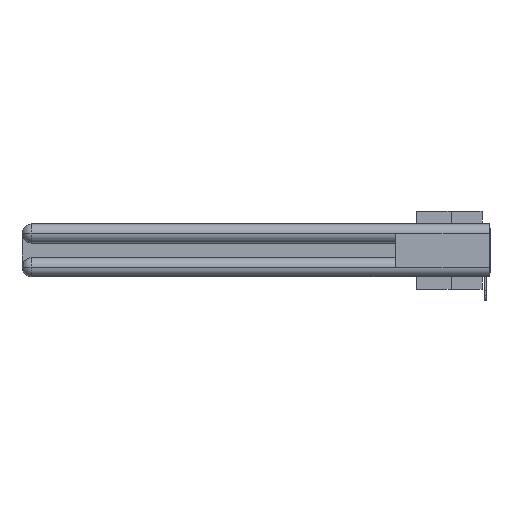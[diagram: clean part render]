
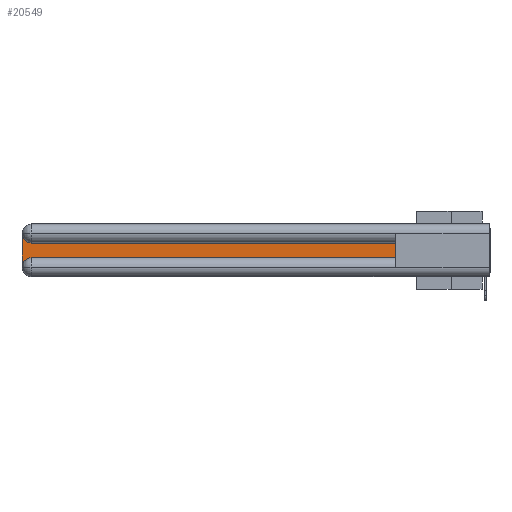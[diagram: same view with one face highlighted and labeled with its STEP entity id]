
A CAD part, left-side view. The second image highlights one B-rep face of the part: STEP entity #20549.
In plain terms, the highlighted planar face has unit normal (-1, 0, 0).
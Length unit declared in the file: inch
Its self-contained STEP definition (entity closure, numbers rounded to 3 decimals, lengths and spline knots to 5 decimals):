
#40 = ORIENTED_EDGE ( 'NONE', *, *, #15962, .T. ) ;
#512 = ORIENTED_EDGE ( 'NONE', *, *, #20141, .T. ) ;
#1826 = VECTOR ( 'NONE', #13648, 39.37008 ) ;
#1877 = DIRECTION ( 'NONE',  ( 1., 0., 0. ) ) ;
#3248 = ORIENTED_EDGE ( 'NONE', *, *, #32857, .T. ) ;
#4267 = VERTEX_POINT ( 'NONE', #34073 ) ;
#5395 = VERTEX_POINT ( 'NONE', #25732 ) ;
#6760 = VECTOR ( 'NONE', #33161, 39.37008 ) ;
#7041 = CARTESIAN_POINT ( 'NONE',  ( 0.075, 0.6, -0.2175 ) ) ;
#7051 = DIRECTION ( 'NONE',  ( 0., -1., 0. ) ) ;
#7186 = CARTESIAN_POINT ( 'NONE',  ( 0.075, 2.94, -0.0625 ) ) ;
#7679 = CARTESIAN_POINT ( 'NONE',  ( 0.075, 2.94, -0.1225 ) ) ;
#9312 = FACE_OUTER_BOUND ( 'NONE', #15956, .T. ) ;
#9491 = DIRECTION ( 'NONE',  ( 1., 0., 0. ) ) ;
#10404 = VECTOR ( 'NONE', #7051, 39.37008 ) ;
#10485 = AXIS2_PLACEMENT_3D ( 'NONE', #7186, #28035, #20163 ) ;
#11069 = EDGE_CURVE ( 'NONE', #18646, #5395, #17308, .T. ) ;
#13648 = DIRECTION ( 'NONE',  ( 0., 0., -1. ) ) ;
#15139 = CARTESIAN_POINT ( 'NONE',  ( 0.075, 3., -0.1225 ) ) ;
#15451 = VERTEX_POINT ( 'NONE', #31141 ) ;
#15563 = ORIENTED_EDGE ( 'NONE', *, *, #25791, .T. ) ;
#15956 = EDGE_LOOP ( 'NONE', ( #40, #26945, #512, #24864, #15563, #3248 ) ) ;
#15962 = EDGE_CURVE ( 'NONE', #15451, #18646, #18774, .T. ) ;
#17091 = CARTESIAN_POINT ( 'NONE',  ( 0.075, 3., -0.2775 ) ) ;
#17308 = CIRCLE ( 'NONE', #10485, 0.06 ) ;
#17358 = AXIS2_PLACEMENT_3D ( 'NONE', #15139, #1877, #26023 ) ;
#18629 = CARTESIAN_POINT ( 'NONE',  ( 0.075, 3., -0.2175 ) ) ;
#18646 = VERTEX_POINT ( 'NONE', #7679 ) ;
#18774 = LINE ( 'NONE', #28077, #30385 ) ;
#18946 = AXIS2_PLACEMENT_3D ( 'NONE', #25382, #9491, #30683 ) ;
#20141 = EDGE_CURVE ( 'NONE', #5395, #33475, #23021, .T. ) ;
#20163 = DIRECTION ( 'NONE',  ( 0., 0., -1. ) ) ;
#20549 = ADVANCED_FACE ( 'NONE', ( #9312 ), #31017, .F. ) ;
#23021 = LINE ( 'NONE', #18629, #1826 ) ;
#23280 = CARTESIAN_POINT ( 'NONE',  ( 0.075, 0.6, -0.2175 ) ) ;
#23400 = EDGE_CURVE ( 'NONE', #33475, #32467, #31752, .T. ) ;
#24864 = ORIENTED_EDGE ( 'NONE', *, *, #23400, .T. ) ;
#25382 = CARTESIAN_POINT ( 'NONE',  ( 0.075, 2.94, -0.2775 ) ) ;
#25732 = CARTESIAN_POINT ( 'NONE',  ( 0.075, 3., -0.0625 ) ) ;
#25791 = EDGE_CURVE ( 'NONE', #32467, #4267, #27818, .T. ) ;
#26023 = DIRECTION ( 'NONE',  ( 0., 0., -1. ) ) ;
#26945 = ORIENTED_EDGE ( 'NONE', *, *, #11069, .T. ) ;
#27818 = LINE ( 'NONE', #23280, #10404 ) ;
#28035 = DIRECTION ( 'NONE',  ( 1., 0., 0. ) ) ;
#28077 = CARTESIAN_POINT ( 'NONE',  ( 0.075, 0.6, -0.1225 ) ) ;
#30385 = VECTOR ( 'NONE', #33713, 39.37008 ) ;
#30683 = DIRECTION ( 'NONE',  ( 0., 0., -1. ) ) ;
#31017 = PLANE ( 'NONE',  #17358 ) ;
#31141 = CARTESIAN_POINT ( 'NONE',  ( 0.075, 0.6, -0.1225 ) ) ;
#31752 = CIRCLE ( 'NONE', #18946, 0.06 ) ;
#32467 = VERTEX_POINT ( 'NONE', #34144 ) ;
#32495 = LINE ( 'NONE', #7041, #6760 ) ;
#32857 = EDGE_CURVE ( 'NONE', #4267, #15451, #32495, .T. ) ;
#33161 = DIRECTION ( 'NONE',  ( 0., 0., 1. ) ) ;
#33475 = VERTEX_POINT ( 'NONE', #17091 ) ;
#33713 = DIRECTION ( 'NONE',  ( 0., 1., 0. ) ) ;
#34073 = CARTESIAN_POINT ( 'NONE',  ( 0.075, 0.6, -0.2175 ) ) ;
#34144 = CARTESIAN_POINT ( 'NONE',  ( 0.075, 2.94, -0.2175 ) ) ;
